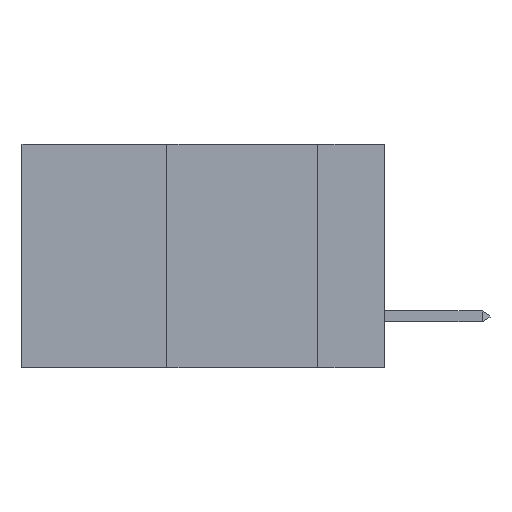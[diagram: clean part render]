
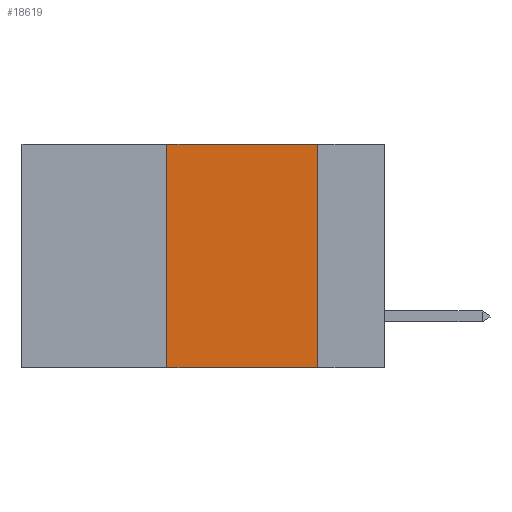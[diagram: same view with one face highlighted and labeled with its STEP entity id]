
A CAD part, left-side view. The second image highlights one B-rep face of the part: STEP entity #18619.
In plain terms, the highlighted planar face has unit normal (-1, 0, 0).
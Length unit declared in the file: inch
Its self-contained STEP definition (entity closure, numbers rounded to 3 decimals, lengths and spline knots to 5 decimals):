
#428 = DIRECTION ( 'NONE',  ( 1., 0., 0. ) ) ;
#679 = ORIENTED_EDGE ( 'NONE', *, *, #1015, .F. ) ;
#1015 = EDGE_CURVE ( 'NONE', #6420, #10804, #19705, .T. ) ;
#1157 = EDGE_CURVE ( 'NONE', #9849, #6420, #7504, .T. ) ;
#1240 = DIRECTION ( 'NONE',  ( 0., 0., -1. ) ) ;
#1373 = CARTESIAN_POINT ( 'NONE',  ( 0., 0.11, 0. ) ) ;
#2857 = CARTESIAN_POINT ( 'NONE',  ( 0., 0.36, 0. ) ) ;
#3125 = ORIENTED_EDGE ( 'NONE', *, *, #18900, .T. ) ;
#3392 = CARTESIAN_POINT ( 'NONE',  ( 0., 0.11, -0.37 ) ) ;
#3591 = VECTOR ( 'NONE', #7257, 39.37008 ) ;
#4946 = LINE ( 'NONE', #7162, #13973 ) ;
#5061 = CARTESIAN_POINT ( 'NONE',  ( 0., 0.11, 0. ) ) ;
#6420 = VERTEX_POINT ( 'NONE', #5061 ) ;
#7162 = CARTESIAN_POINT ( 'NONE',  ( 0., 0.36, 0. ) ) ;
#7257 = DIRECTION ( 'NONE',  ( 0., -1., 0. ) ) ;
#7461 = AXIS2_PLACEMENT_3D ( 'NONE', #11518, #428, #13303 ) ;
#7504 = LINE ( 'NONE', #17265, #16438 ) ;
#8426 = VERTEX_POINT ( 'NONE', #14826 ) ;
#8974 = DIRECTION ( 'NONE',  ( 0., 0., 1. ) ) ;
#9381 = EDGE_LOOP ( 'NONE', ( #679, #11148, #11411, #3125 ) ) ;
#9849 = VERTEX_POINT ( 'NONE', #2857 ) ;
#10804 = VERTEX_POINT ( 'NONE', #3392 ) ;
#11148 = ORIENTED_EDGE ( 'NONE', *, *, #1157, .F. ) ;
#11236 = DIRECTION ( 'NONE',  ( 0., -1., 0. ) ) ;
#11411 = ORIENTED_EDGE ( 'NONE', *, *, #21181, .F. ) ;
#11518 = CARTESIAN_POINT ( 'NONE',  ( 0., 0.6, 0. ) ) ;
#13220 = PLANE ( 'NONE',  #7461 ) ;
#13303 = DIRECTION ( 'NONE',  ( 0., 0., -1. ) ) ;
#13973 = VECTOR ( 'NONE', #8974, 39.37008 ) ;
#14515 = VECTOR ( 'NONE', #1240, 39.37008 ) ;
#14826 = CARTESIAN_POINT ( 'NONE',  ( 0., 0.36, -0.37 ) ) ;
#14904 = FACE_OUTER_BOUND ( 'NONE', #9381, .T. ) ;
#16171 = CARTESIAN_POINT ( 'NONE',  ( 0., 0.6, -0.37 ) ) ;
#16438 = VECTOR ( 'NONE', #11236, 39.37008 ) ;
#17265 = CARTESIAN_POINT ( 'NONE',  ( 0., 0.6, 0. ) ) ;
#18478 = LINE ( 'NONE', #16171, #3591 ) ;
#18619 = ADVANCED_FACE ( 'NONE', ( #14904 ), #13220, .F. ) ;
#18900 = EDGE_CURVE ( 'NONE', #8426, #10804, #18478, .T. ) ;
#19705 = LINE ( 'NONE', #1373, #14515 ) ;
#21181 = EDGE_CURVE ( 'NONE', #8426, #9849, #4946, .T. ) ;
